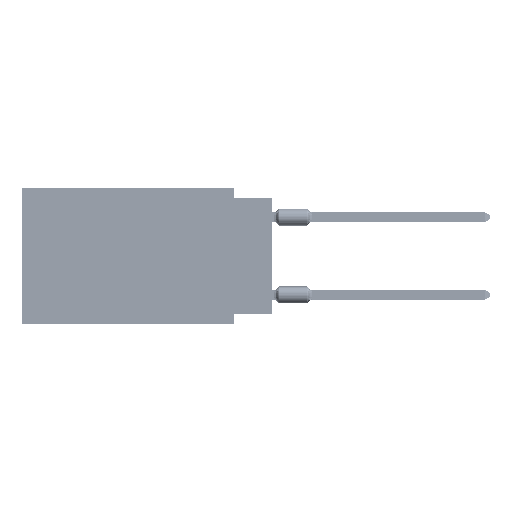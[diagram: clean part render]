
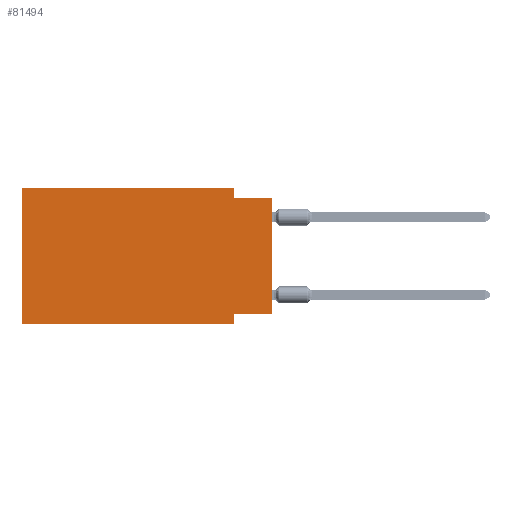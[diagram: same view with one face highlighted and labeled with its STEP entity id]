
A CAD part, left-side view. The second image highlights one B-rep face of the part: STEP entity #81494.
In plain terms, the highlighted planar face has unit normal (-1, 0, 0).
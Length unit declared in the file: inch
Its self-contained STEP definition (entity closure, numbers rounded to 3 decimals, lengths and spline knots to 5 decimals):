
#2341 = DIRECTION ( 'NONE',  ( 0., 0., 1. ) ) ;
#2921 = LINE ( 'NONE', #110993, #69649 ) ;
#3862 = EDGE_CURVE ( 'NONE', #113885, #112590, #117142, .T. ) ;
#4814 = CARTESIAN_POINT ( 'NONE',  ( 0., 0.1, -0.025 ) ) ;
#5569 = CARTESIAN_POINT ( 'NONE',  ( 0., 0.1, -0.325 ) ) ;
#7028 = CARTESIAN_POINT ( 'NONE',  ( 0., 0., -0.025 ) ) ;
#8387 = CARTESIAN_POINT ( 'NONE',  ( 0., 0.1, 0. ) ) ;
#8486 = CARTESIAN_POINT ( 'NONE',  ( 0., 0., -0.325 ) ) ;
#13685 = DIRECTION ( 'NONE',  ( 0., -1., 0. ) ) ;
#15170 = ORIENTED_EDGE ( 'NONE', *, *, #25174, .T. ) ;
#17493 = VERTEX_POINT ( 'NONE', #39893 ) ;
#17503 = LINE ( 'NONE', #8486, #71928 ) ;
#18614 = DIRECTION ( 'NONE',  ( 0., 0., 1. ) ) ;
#20379 = ORIENTED_EDGE ( 'NONE', *, *, #109588, .F. ) ;
#21655 = VECTOR ( 'NONE', #18614, 39.37008 ) ;
#25174 = EDGE_CURVE ( 'NONE', #33872, #17493, #114542, .T. ) ;
#25859 = CARTESIAN_POINT ( 'NONE',  ( 0., 0., -0.025 ) ) ;
#27617 = LINE ( 'NONE', #54655, #21655 ) ;
#28948 = VERTEX_POINT ( 'NONE', #5569 ) ;
#29704 = PLANE ( 'NONE',  #91076 ) ;
#33370 = CARTESIAN_POINT ( 'NONE',  ( 0., 0., -0.325 ) ) ;
#33872 = VERTEX_POINT ( 'NONE', #55076 ) ;
#35227 = ORIENTED_EDGE ( 'NONE', *, *, #90326, .F. ) ;
#38728 = DIRECTION ( 'NONE',  ( 0., 0., -1. ) ) ;
#39893 = CARTESIAN_POINT ( 'NONE',  ( 0., 0.1, -0.35 ) ) ;
#42412 = EDGE_CURVE ( 'NONE', #59361, #101812, #68263, .T. ) ;
#45014 = DIRECTION ( 'NONE',  ( 0., 0., -1. ) ) ;
#46725 = VECTOR ( 'NONE', #52683, 39.37008 ) ;
#47894 = EDGE_CURVE ( 'NONE', #108569, #28948, #17503, .T. ) ;
#49075 = ORIENTED_EDGE ( 'NONE', *, *, #42412, .F. ) ;
#52683 = DIRECTION ( 'NONE',  ( 0., 0., -1. ) ) ;
#53271 = CARTESIAN_POINT ( 'NONE',  ( 0., 0.1, -0.35 ) ) ;
#54655 = CARTESIAN_POINT ( 'NONE',  ( 0., 0.645, 0. ) ) ;
#55076 = CARTESIAN_POINT ( 'NONE',  ( 0., 0.645, -0.35 ) ) ;
#59361 = VERTEX_POINT ( 'NONE', #88119 ) ;
#66504 = CARTESIAN_POINT ( 'NONE',  ( 0., 0.645, 0. ) ) ;
#68263 = LINE ( 'NONE', #66504, #118684 ) ;
#68444 = CARTESIAN_POINT ( 'NONE',  ( 0., 0.1, 0. ) ) ;
#69116 = DIRECTION ( 'NONE',  ( 0., -1., 0. ) ) ;
#69649 = VECTOR ( 'NONE', #2341, 39.37008 ) ;
#71928 = VECTOR ( 'NONE', #100329, 39.37008 ) ;
#74139 = FACE_OUTER_BOUND ( 'NONE', #85498, .T. ) ;
#79250 = EDGE_CURVE ( 'NONE', #108569, #112590, #2921, .T. ) ;
#81494 = ADVANCED_FACE ( 'NONE', ( #74139 ), #29704, .F. ) ;
#81544 = ORIENTED_EDGE ( 'NONE', *, *, #79250, .T. ) ;
#81658 = ORIENTED_EDGE ( 'NONE', *, *, #99369, .F. ) ;
#83283 = ORIENTED_EDGE ( 'NONE', *, *, #47894, .F. ) ;
#85498 = EDGE_LOOP ( 'NONE', ( #81544, #93076, #35227, #49075, #20379, #15170, #81658, #83283 ) ) ;
#88119 = CARTESIAN_POINT ( 'NONE',  ( 0., 0.645, 0. ) ) ;
#90326 = EDGE_CURVE ( 'NONE', #101812, #113885, #90628, .T. ) ;
#90628 = LINE ( 'NONE', #8387, #97986 ) ;
#91076 = AXIS2_PLACEMENT_3D ( 'NONE', #110771, #111377, #38728 ) ;
#92924 = DIRECTION ( 'NONE',  ( 0., -1., 0. ) ) ;
#93076 = ORIENTED_EDGE ( 'NONE', *, *, #3862, .F. ) ;
#95933 = CARTESIAN_POINT ( 'NONE',  ( 0., 0.645, -0.35 ) ) ;
#97986 = VECTOR ( 'NONE', #45014, 39.37008 ) ;
#98314 = LINE ( 'NONE', #53271, #46725 ) ;
#99369 = EDGE_CURVE ( 'NONE', #28948, #17493, #98314, .T. ) ;
#100095 = VECTOR ( 'NONE', #13685, 39.37008 ) ;
#100329 = DIRECTION ( 'NONE',  ( 0., 1., 0. ) ) ;
#101460 = VECTOR ( 'NONE', #69116, 39.37008 ) ;
#101812 = VERTEX_POINT ( 'NONE', #68444 ) ;
#108569 = VERTEX_POINT ( 'NONE', #33370 ) ;
#109588 = EDGE_CURVE ( 'NONE', #33872, #59361, #27617, .T. ) ;
#110771 = CARTESIAN_POINT ( 'NONE',  ( 0., 0.645, 0. ) ) ;
#110993 = CARTESIAN_POINT ( 'NONE',  ( 0., 0., 0. ) ) ;
#111377 = DIRECTION ( 'NONE',  ( 1., 0., 0. ) ) ;
#112590 = VERTEX_POINT ( 'NONE', #7028 ) ;
#113885 = VERTEX_POINT ( 'NONE', #4814 ) ;
#114542 = LINE ( 'NONE', #95933, #100095 ) ;
#117142 = LINE ( 'NONE', #25859, #101460 ) ;
#118684 = VECTOR ( 'NONE', #92924, 39.37008 ) ;
